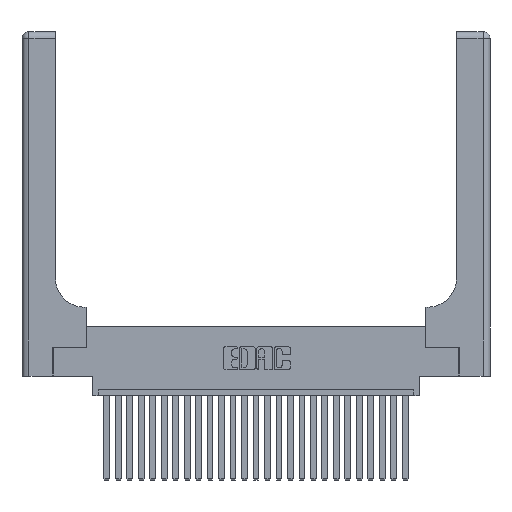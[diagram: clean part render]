
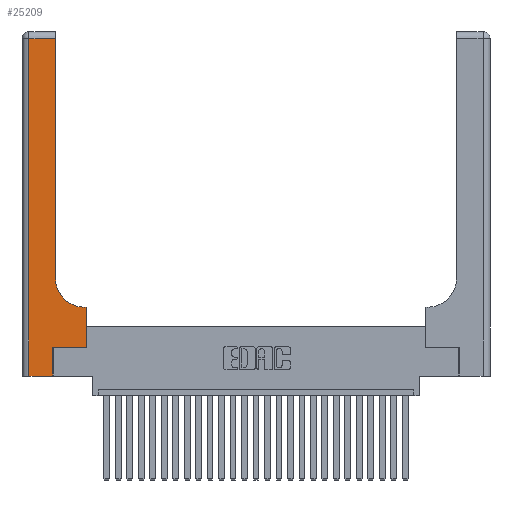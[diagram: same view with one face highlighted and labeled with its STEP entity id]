
A CAD part, top view. The second image highlights one B-rep face of the part: STEP entity #25209.
In plain terms, the highlighted planar face has unit normal (0, 0, 1).
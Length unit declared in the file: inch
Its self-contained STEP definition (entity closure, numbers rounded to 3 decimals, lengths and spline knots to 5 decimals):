
#366 = ORIENTED_EDGE ( 'NONE', *, *, #1492, .T. ) ;
#483 = AXIS2_PLACEMENT_3D ( 'NONE', #17375, #11326, #840 ) ;
#553 = ORIENTED_EDGE ( 'NONE', *, *, #17305, .T. ) ;
#840 = DIRECTION ( 'NONE',  ( 1., 0., 0. ) ) ;
#1164 = VECTOR ( 'NONE', #10420, 39.37008 ) ;
#1492 = EDGE_CURVE ( 'NONE', #27411, #18845, #12478, .T. ) ;
#1668 = ORIENTED_EDGE ( 'NONE', *, *, #7008, .T. ) ;
#1733 = CARTESIAN_POINT ( 'NONE',  ( 0., 2.94, 0.37 ) ) ;
#1763 = CARTESIAN_POINT ( 'NONE',  ( 0.5585, 0.25, 0.37 ) ) ;
#2588 = VERTEX_POINT ( 'NONE', #8677 ) ;
#3937 = VERTEX_POINT ( 'NONE', #5428 ) ;
#4006 = LINE ( 'NONE', #1733, #14254 ) ;
#4755 = DIRECTION ( 'NONE',  ( -1., 0., 0. ) ) ;
#4786 = VERTEX_POINT ( 'NONE', #9225 ) ;
#5428 = CARTESIAN_POINT ( 'NONE',  ( 0.269, 0., 0.37 ) ) ;
#5747 = CARTESIAN_POINT ( 'NONE',  ( 0.2915, 0.85, 0.37 ) ) ;
#5880 = CARTESIAN_POINT ( 'NONE',  ( 0.5415, 0.6, 0.37 ) ) ;
#6314 = LINE ( 'NONE', #17740, #8698 ) ;
#7008 = EDGE_CURVE ( 'NONE', #18845, #4786, #4006, .T. ) ;
#7166 = EDGE_LOOP ( 'NONE', ( #366, #1668, #26846, #24257, #16060, #18707, #18055, #21285, #553 ) ) ;
#8052 = DIRECTION ( 'NONE',  ( 0., 1., 0. ) ) ;
#8677 = CARTESIAN_POINT ( 'NONE',  ( 0.269, 0.25, 0.37 ) ) ;
#8698 = VECTOR ( 'NONE', #19791, 39.37008 ) ;
#9191 = VECTOR ( 'NONE', #14763, 39.37008 ) ;
#9225 = CARTESIAN_POINT ( 'NONE',  ( 0.06, 2.94, 0.37 ) ) ;
#9576 = VERTEX_POINT ( 'NONE', #1763 ) ;
#10420 = DIRECTION ( 'NONE',  ( 0., -1., 0. ) ) ;
#11326 = DIRECTION ( 'NONE',  ( 0., 0., -1. ) ) ;
#11980 = VECTOR ( 'NONE', #8052, 39.37008 ) ;
#12478 = LINE ( 'NONE', #12708, #9191 ) ;
#12656 = CARTESIAN_POINT ( 'NONE',  ( 0., 0., 0.37 ) ) ;
#12708 = CARTESIAN_POINT ( 'NONE',  ( 0.2915, 3., 0.37 ) ) ;
#12800 = LINE ( 'NONE', #20907, #1164 ) ;
#13038 = EDGE_CURVE ( 'NONE', #9576, #17019, #17644, .T. ) ;
#13182 = CARTESIAN_POINT ( 'NONE',  ( 0.2915, 0.6, 0.37 ) ) ;
#13367 = DIRECTION ( 'NONE',  ( 0., 0., -1. ) ) ;
#14254 = VECTOR ( 'NONE', #25215, 39.37008 ) ;
#14763 = DIRECTION ( 'NONE',  ( 0., 1., 0. ) ) ;
#14784 = CARTESIAN_POINT ( 'NONE',  ( 0.269, 0., 0.37 ) ) ;
#14891 = VERTEX_POINT ( 'NONE', #5880 ) ;
#15259 = CARTESIAN_POINT ( 'NONE',  ( 0.2915, 2.94, 0.37 ) ) ;
#15343 = EDGE_CURVE ( 'NONE', #4786, #20672, #12800, .T. ) ;
#15861 = EDGE_CURVE ( 'NONE', #17019, #14891, #25257, .T. ) ;
#15946 = VECTOR ( 'NONE', #4755, 39.37008 ) ;
#16060 = ORIENTED_EDGE ( 'NONE', *, *, #26883, .T. ) ;
#16748 = DIRECTION ( 'NONE',  ( 0., 1., 0. ) ) ;
#16956 = EDGE_CURVE ( 'NONE', #20672, #3937, #25888, .T. ) ;
#17019 = VERTEX_POINT ( 'NONE', #21601 ) ;
#17305 = EDGE_CURVE ( 'NONE', #14891, #27411, #22189, .T. ) ;
#17375 = CARTESIAN_POINT ( 'NONE',  ( 0.5415, 0.85, 0.37 ) ) ;
#17644 = LINE ( 'NONE', #18908, #11980 ) ;
#17740 = CARTESIAN_POINT ( 'NONE',  ( 0.269, 0.25, 0.37 ) ) ;
#18055 = ORIENTED_EDGE ( 'NONE', *, *, #13038, .T. ) ;
#18707 = ORIENTED_EDGE ( 'NONE', *, *, #20594, .T. ) ;
#18845 = VERTEX_POINT ( 'NONE', #15259 ) ;
#18908 = CARTESIAN_POINT ( 'NONE',  ( 0.5585, 0.25, 0.37 ) ) ;
#19270 = DIRECTION ( 'NONE',  ( 1., 0., 0. ) ) ;
#19450 = DIRECTION ( 'NONE',  ( -1., 0., 0. ) ) ;
#19626 = AXIS2_PLACEMENT_3D ( 'NONE', #25765, #13367, #19450 ) ;
#19791 = DIRECTION ( 'NONE',  ( 1., 0., 0. ) ) ;
#20056 = FACE_OUTER_BOUND ( 'NONE', #7166, .T. ) ;
#20594 = EDGE_CURVE ( 'NONE', #2588, #9576, #6314, .T. ) ;
#20672 = VERTEX_POINT ( 'NONE', #22009 ) ;
#20907 = CARTESIAN_POINT ( 'NONE',  ( 0.06, 3., 0.37 ) ) ;
#21285 = ORIENTED_EDGE ( 'NONE', *, *, #15861, .T. ) ;
#21601 = CARTESIAN_POINT ( 'NONE',  ( 0.5585, 0.6, 0.37 ) ) ;
#22009 = CARTESIAN_POINT ( 'NONE',  ( 0.06, 0., 0.37 ) ) ;
#22110 = LINE ( 'NONE', #14784, #25776 ) ;
#22189 = CIRCLE ( 'NONE', #483, 0.25 ) ;
#23618 = PLANE ( 'NONE',  #19626 ) ;
#24257 = ORIENTED_EDGE ( 'NONE', *, *, #16956, .T. ) ;
#25209 = ADVANCED_FACE ( 'NONE', ( #20056 ), #23618, .F. ) ;
#25215 = DIRECTION ( 'NONE',  ( -1., 0., 0. ) ) ;
#25257 = LINE ( 'NONE', #13182, #15946 ) ;
#25765 = CARTESIAN_POINT ( 'NONE',  ( 0., 3., 0.37 ) ) ;
#25776 = VECTOR ( 'NONE', #16748, 39.37008 ) ;
#25888 = LINE ( 'NONE', #12656, #26192 ) ;
#26192 = VECTOR ( 'NONE', #19270, 39.37008 ) ;
#26846 = ORIENTED_EDGE ( 'NONE', *, *, #15343, .T. ) ;
#26883 = EDGE_CURVE ( 'NONE', #3937, #2588, #22110, .T. ) ;
#27411 = VERTEX_POINT ( 'NONE', #5747 ) ;
